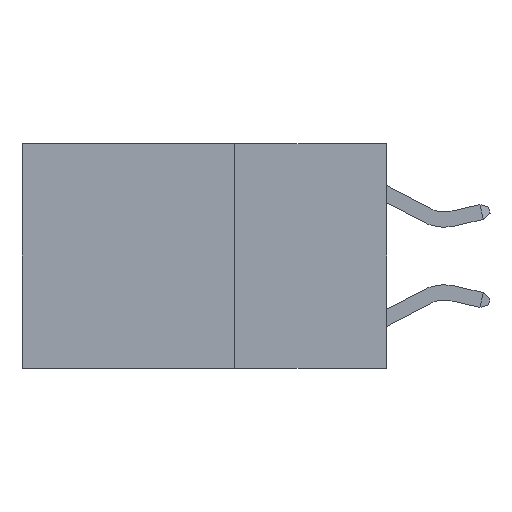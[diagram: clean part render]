
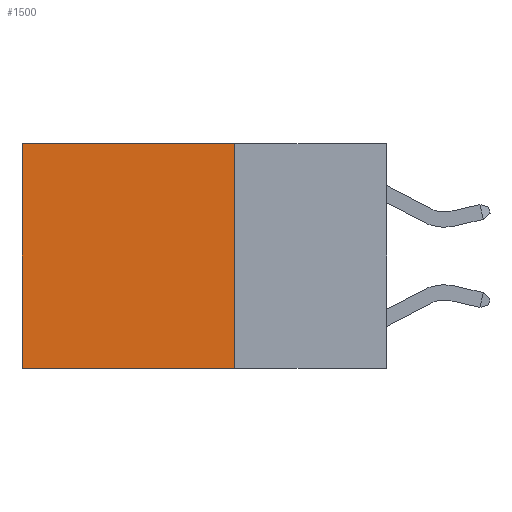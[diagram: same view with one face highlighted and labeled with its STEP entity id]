
A CAD part, left-side view. The second image highlights one B-rep face of the part: STEP entity #1500.
In plain terms, the highlighted planar face has unit normal (-1, 0, 0).
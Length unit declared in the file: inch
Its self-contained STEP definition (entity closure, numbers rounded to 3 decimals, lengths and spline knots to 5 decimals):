
#72 = CARTESIAN_POINT ( 'NONE',  ( 0.2625, 0.6, -0.37 ) ) ;
#88 = LINE ( 'NONE', #13372, #4584 ) ;
#1076 = VECTOR ( 'NONE', #9124, 39.37008 ) ;
#1500 = ADVANCED_FACE ( 'NONE', ( #6618 ), #11034, .F. ) ;
#1723 = EDGE_CURVE ( 'NONE', #5899, #11170, #9746, .T. ) ;
#1852 = DIRECTION ( 'NONE',  ( 0., 1., 0. ) ) ;
#3074 = CARTESIAN_POINT ( 'NONE',  ( 0.2625, 0.25, 0. ) ) ;
#3383 = DIRECTION ( 'NONE',  ( 0., 0., -1. ) ) ;
#3438 = DIRECTION ( 'NONE',  ( 1., 0., 0. ) ) ;
#4528 = EDGE_CURVE ( 'NONE', #11170, #7244, #6434, .T. ) ;
#4584 = VECTOR ( 'NONE', #3383, 39.37008 ) ;
#4741 = VECTOR ( 'NONE', #1852, 39.37008 ) ;
#5289 = AXIS2_PLACEMENT_3D ( 'NONE', #10320, #3438, #12455 ) ;
#5445 = EDGE_CURVE ( 'NONE', #5899, #13755, #8293, .T. ) ;
#5899 = VERTEX_POINT ( 'NONE', #7092 ) ;
#6434 = LINE ( 'NONE', #9461, #4741 ) ;
#6618 = FACE_OUTER_BOUND ( 'NONE', #14113, .T. ) ;
#6745 = ORIENTED_EDGE ( 'NONE', *, *, #1723, .F. ) ;
#6761 = CARTESIAN_POINT ( 'NONE',  ( 0.2625, 0.25, -0.37 ) ) ;
#6859 = EDGE_CURVE ( 'NONE', #13755, #7244, #88, .T. ) ;
#7092 = CARTESIAN_POINT ( 'NONE',  ( 0.2625, 0.25, 0. ) ) ;
#7155 = ORIENTED_EDGE ( 'NONE', *, *, #5445, .T. ) ;
#7160 = CARTESIAN_POINT ( 'NONE',  ( 0.2625, 0.25, 0. ) ) ;
#7244 = VERTEX_POINT ( 'NONE', #72 ) ;
#7581 = CARTESIAN_POINT ( 'NONE',  ( 0.2625, 0.6, 0. ) ) ;
#8293 = LINE ( 'NONE', #7160, #1076 ) ;
#8408 = ORIENTED_EDGE ( 'NONE', *, *, #6859, .T. ) ;
#9124 = DIRECTION ( 'NONE',  ( 0., 1., 0. ) ) ;
#9461 = CARTESIAN_POINT ( 'NONE',  ( 0.2625, 0.25, -0.37 ) ) ;
#9662 = DIRECTION ( 'NONE',  ( 0., 0., -1. ) ) ;
#9746 = LINE ( 'NONE', #3074, #9810 ) ;
#9810 = VECTOR ( 'NONE', #9662, 39.37008 ) ;
#10320 = CARTESIAN_POINT ( 'NONE',  ( 0.2625, 0.25, 0. ) ) ;
#11034 = PLANE ( 'NONE',  #5289 ) ;
#11170 = VERTEX_POINT ( 'NONE', #6761 ) ;
#11596 = ORIENTED_EDGE ( 'NONE', *, *, #4528, .F. ) ;
#12455 = DIRECTION ( 'NONE',  ( 0., 0., -1. ) ) ;
#13372 = CARTESIAN_POINT ( 'NONE',  ( 0.2625, 0.6, 0. ) ) ;
#13755 = VERTEX_POINT ( 'NONE', #7581 ) ;
#14113 = EDGE_LOOP ( 'NONE', ( #8408, #11596, #6745, #7155 ) ) ;
